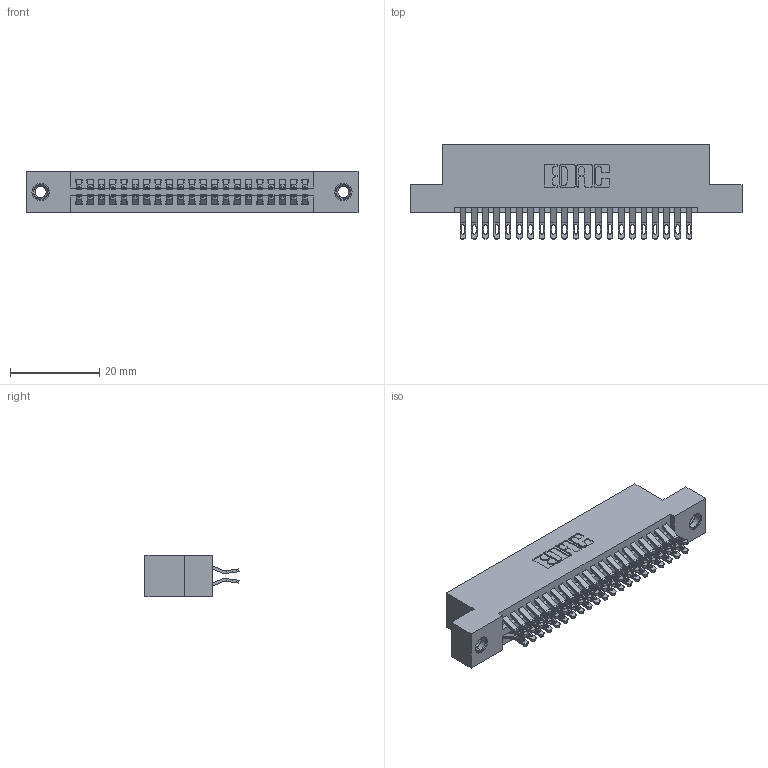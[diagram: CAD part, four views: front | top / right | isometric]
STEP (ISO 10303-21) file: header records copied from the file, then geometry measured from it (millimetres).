
FILE_DESCRIPTION (( 'STEP AP203' ), '1' );
FILE_NAME ('395-042-555-207.STEP', '2018-11-15T11:56:29', ( '' ), ( '' ), 'SwSTEP 2.0', 'SolidWorks 2016', '' );
FILE_SCHEMA (( 'CONFIG_CONTROL_DESIGN' ));
Length unit declared in the file: inch
Products named in the file (4): 345-250-001_345-250-005-103; 345 Part_Flush Mounting Lugs - 0.156 Dia-TI; 345-292-001_555 Tail; 395-042-555-207
Assembly tree (45 placements, depth 2):
  395-042-555-207
    345 Part_Flush Mounting Lugs - 0.156 Dia-TI
    345-292-001_555 Tail  x42
    345-250-001_345-250-005-103  x2
Bounding box: 74.55 x 21.13 x 9.4 mm (x, y, z)
Volume: 7155.1 mm3; surface area: 10621.4 mm2
Topology: 45 solids, 45 shells, 2538 faces, 7911 edges, 5266 vertices
Faces by surface type: plane 1414, cylinder 1108, cone 12, torus 4
Entity records: 20816 total; most frequent: CARTESIAN_POINT 3525, ORIENTED_EDGE 3422, DIRECTION 3129, EDGE_CURVE 1711, VECTOR 1455, LINE 1455, VERTEX_POINT 1136, AXIS2_PLACEMENT_3D 837
